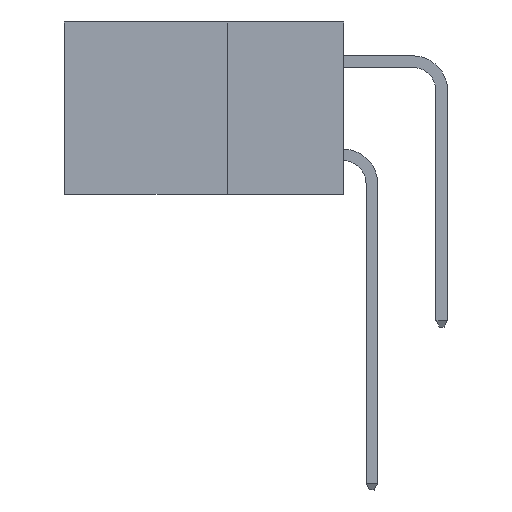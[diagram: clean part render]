
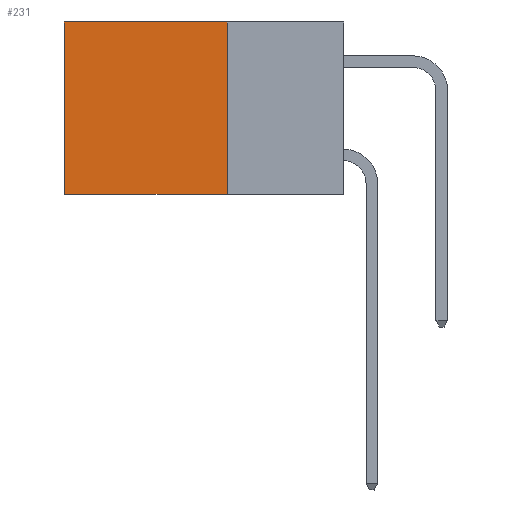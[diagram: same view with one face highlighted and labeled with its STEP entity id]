
A CAD part, left-side view. The second image highlights one B-rep face of the part: STEP entity #231.
In plain terms, the highlighted planar face has unit normal (-1, 0, 0).
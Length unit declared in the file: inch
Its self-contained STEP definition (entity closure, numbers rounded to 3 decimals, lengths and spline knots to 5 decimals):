
#231 = ADVANCED_FACE ( 'NONE', ( #1338 ), #12914, .F. ) ;
#234 = EDGE_CURVE ( 'NONE', #8377, #7981, #2417, .T. ) ;
#596 = CARTESIAN_POINT ( 'NONE',  ( 0.2615, 0.6, -0.37 ) ) ;
#1338 = FACE_OUTER_BOUND ( 'NONE', #3842, .T. ) ;
#1591 = LINE ( 'NONE', #4891, #5303 ) ;
#2313 = CARTESIAN_POINT ( 'NONE',  ( 0.2615, 0.25, 0. ) ) ;
#2417 = LINE ( 'NONE', #4950, #5877 ) ;
#3339 = CARTESIAN_POINT ( 'NONE',  ( 0.2615, 0.25, 0. ) ) ;
#3842 = EDGE_LOOP ( 'NONE', ( #9144, #10407, #6674, #12286 ) ) ;
#4891 = CARTESIAN_POINT ( 'NONE',  ( 0.2615, 0.25, -0.37 ) ) ;
#4950 = CARTESIAN_POINT ( 'NONE',  ( 0.2615, 0.25, -0.37 ) ) ;
#5255 = DIRECTION ( 'NONE',  ( 0., 0., -1. ) ) ;
#5303 = VECTOR ( 'NONE', #13087, 39.37008 ) ;
#5757 = VECTOR ( 'NONE', #12693, 39.37008 ) ;
#5877 = VECTOR ( 'NONE', #7090, 39.37008 ) ;
#6009 = DIRECTION ( 'NONE',  ( 1., 0., 0. ) ) ;
#6674 = ORIENTED_EDGE ( 'NONE', *, *, #234, .F. ) ;
#7090 = DIRECTION ( 'NONE',  ( 0., 0., -1. ) ) ;
#7098 = AXIS2_PLACEMENT_3D ( 'NONE', #9469, #6009, #9397 ) ;
#7981 = VERTEX_POINT ( 'NONE', #8477 ) ;
#8377 = VERTEX_POINT ( 'NONE', #2313 ) ;
#8477 = CARTESIAN_POINT ( 'NONE',  ( 0.2615, 0.25, -0.37 ) ) ;
#9144 = ORIENTED_EDGE ( 'NONE', *, *, #11957, .T. ) ;
#9397 = DIRECTION ( 'NONE',  ( 0., 0., -1. ) ) ;
#9469 = CARTESIAN_POINT ( 'NONE',  ( 0.2615, 0.25, -0.37 ) ) ;
#10407 = ORIENTED_EDGE ( 'NONE', *, *, #13202, .F. ) ;
#11106 = LINE ( 'NONE', #596, #13121 ) ;
#11957 = EDGE_CURVE ( 'NONE', #15025, #12822, #11106, .T. ) ;
#12121 = EDGE_CURVE ( 'NONE', #8377, #15025, #13831, .T. ) ;
#12286 = ORIENTED_EDGE ( 'NONE', *, *, #12121, .T. ) ;
#12493 = CARTESIAN_POINT ( 'NONE',  ( 0.2615, 0.6, -0.37 ) ) ;
#12693 = DIRECTION ( 'NONE',  ( 0., 1., 0. ) ) ;
#12822 = VERTEX_POINT ( 'NONE', #12493 ) ;
#12914 = PLANE ( 'NONE',  #7098 ) ;
#13087 = DIRECTION ( 'NONE',  ( 0., 1., 0. ) ) ;
#13121 = VECTOR ( 'NONE', #5255, 39.37008 ) ;
#13202 = EDGE_CURVE ( 'NONE', #7981, #12822, #1591, .T. ) ;
#13831 = LINE ( 'NONE', #3339, #5757 ) ;
#15006 = CARTESIAN_POINT ( 'NONE',  ( 0.2615, 0.6, 0. ) ) ;
#15025 = VERTEX_POINT ( 'NONE', #15006 ) ;
